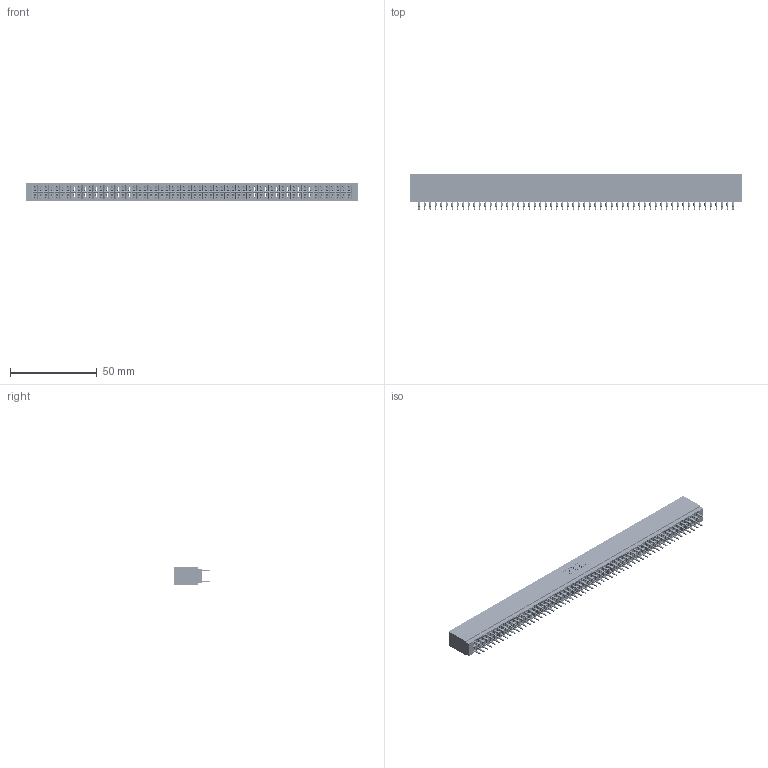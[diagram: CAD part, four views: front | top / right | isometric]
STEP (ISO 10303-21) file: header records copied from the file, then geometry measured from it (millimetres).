
FILE_DESCRIPTION (( 'STEP AP203' ), '1' );
FILE_NAME ('746-116-560-201.STEP', '2026-03-06T16:55:12', ( '' ), ( '' ), 'SwSTEP 2.0', 'SolidWorks 2023', '' );
FILE_SCHEMA (( 'CONFIG_CONTROL_DESIGN' ));
Products named in the file (3): 746-116-560-201; 746 Part_.515 Slot Depth - 01; 746-292-001_560
Assembly tree (117 placements, depth 2):
  746-116-560-201
    746 Part_.515 Slot Depth - 01
    746-292-001_560  x116
Bounding box: 191.39 x 20.82 x 9.91 mm (x, y, z)
Volume: 20813.7 mm3; surface area: 35634.1 mm2
Topology: 117 solids, 117 shells, 11059 faces, 30771 edges, 19721 vertices
Faces by surface type: plane 5507, cylinder 2536, bspline 2320, torus 696
Entity records: 87432 total; most frequent: CARTESIAN_POINT 17239, ORIENTED_EDGE 15082, DIRECTION 12571, EDGE_CURVE 7541, VECTOR 6769, LINE 6769, VERTEX_POINT 5001, AXIS2_PLACEMENT_3D 2901
